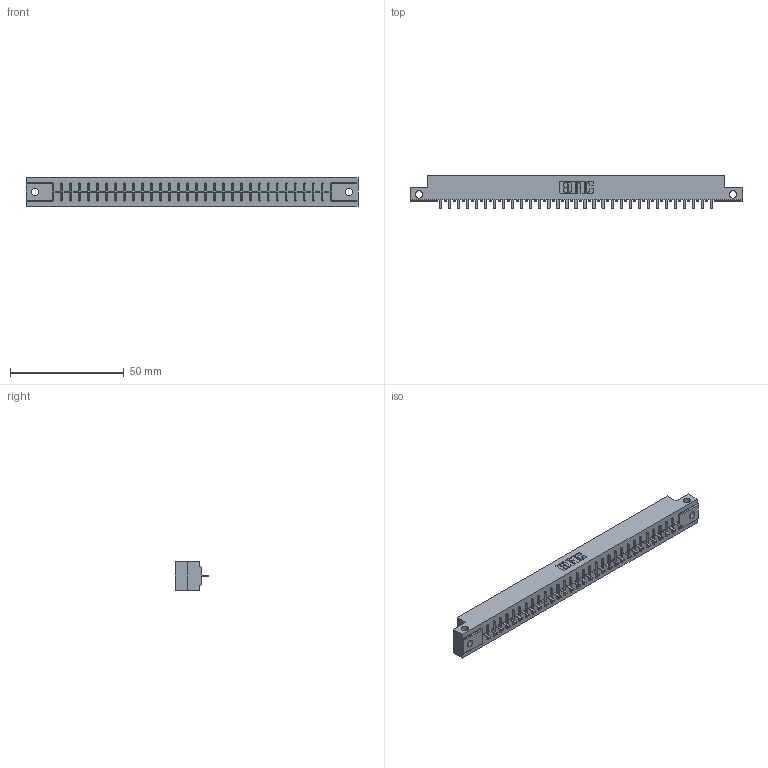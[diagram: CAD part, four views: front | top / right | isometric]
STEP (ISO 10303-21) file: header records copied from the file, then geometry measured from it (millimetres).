
FILE_DESCRIPTION (( 'STEP AP203' ), '1' );
FILE_NAME ('356-031-421-112.STEP', '2020-09-23T21:00:49', ( '' ), ( '' ), 'SwSTEP 2.0', 'SolidWorks 2020', '' );
FILE_SCHEMA (( 'CONFIG_CONTROL_DESIGN' ));
Length unit declared in the file: inch
Products named in the file (3): 306-290-001_121; 306 Part_.128 Dia; 356-031-421-112
Assembly tree (32 placements, depth 2):
  356-031-421-112
    306 Part_.128 Dia
    306-290-001_121  x31
Bounding box: 145.85 x 14.88 x 12.7 mm (x, y, z)
Volume: 15784.4 mm3; surface area: 15895.2 mm2
Topology: 32 solids, 32 shells, 2298 faces, 6459 edges, 4134 vertices
Faces by surface type: plane 1525, cylinder 649, sphere 124
Entity records: 30696 total; most frequent: CARTESIAN_POINT 5200, ORIENTED_EDGE 5110, DIRECTION 5067, EDGE_CURVE 2555, LINE 1977, VECTOR 1977, VERTEX_POINT 1614, AXIS2_PLACEMENT_3D 1545
